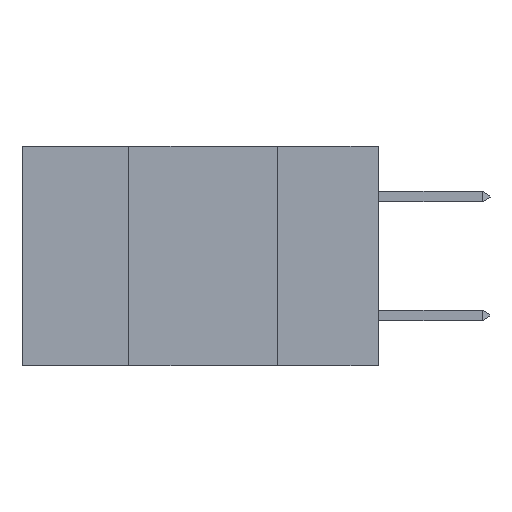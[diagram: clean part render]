
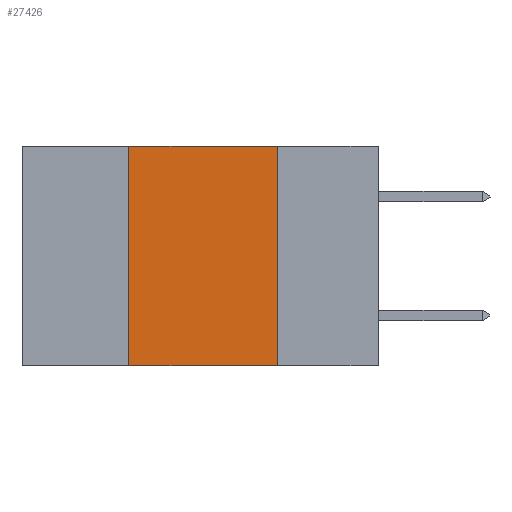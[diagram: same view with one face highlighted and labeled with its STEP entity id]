
A CAD part, left-side view. The second image highlights one B-rep face of the part: STEP entity #27426.
In plain terms, the highlighted planar face has unit normal (-1, 0, 0).
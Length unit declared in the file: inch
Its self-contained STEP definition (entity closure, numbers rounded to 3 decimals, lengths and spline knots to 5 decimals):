
#52 = CARTESIAN_POINT ( 'NONE',  ( 0., 0.17, 0. ) ) ;
#2374 = ORIENTED_EDGE ( 'NONE', *, *, #3231, .F. ) ;
#2716 = VERTEX_POINT ( 'NONE', #6277 ) ;
#2918 = DIRECTION ( 'NONE',  ( 0., -1., 0. ) ) ;
#3231 = EDGE_CURVE ( 'NONE', #17648, #2716, #27970, .T. ) ;
#6277 = CARTESIAN_POINT ( 'NONE',  ( 0., 0.42, 0. ) ) ;
#7443 = PLANE ( 'NONE',  #23308 ) ;
#7758 = EDGE_LOOP ( 'NONE', ( #9917, #26870, #2374, #13722 ) ) ;
#7793 = CARTESIAN_POINT ( 'NONE',  ( 0., 0.6, 0. ) ) ;
#8834 = VECTOR ( 'NONE', #10053, 39.37008 ) ;
#8847 = VECTOR ( 'NONE', #10106, 39.37008 ) ;
#9709 = DIRECTION ( 'NONE',  ( 1., 0., 0. ) ) ;
#9917 = ORIENTED_EDGE ( 'NONE', *, *, #11783, .F. ) ;
#10053 = DIRECTION ( 'NONE',  ( 0., -1., 0. ) ) ;
#10106 = DIRECTION ( 'NONE',  ( 0., 0., -1. ) ) ;
#10343 = DIRECTION ( 'NONE',  ( 0., 0., 1. ) ) ;
#11783 = EDGE_CURVE ( 'NONE', #18381, #17428, #20709, .T. ) ;
#13722 = ORIENTED_EDGE ( 'NONE', *, *, #20954, .T. ) ;
#14723 = LINE ( 'NONE', #25275, #19960 ) ;
#14748 = LINE ( 'NONE', #7793, #8834 ) ;
#17428 = VERTEX_POINT ( 'NONE', #23968 ) ;
#17648 = VERTEX_POINT ( 'NONE', #17990 ) ;
#17990 = CARTESIAN_POINT ( 'NONE',  ( 0., 0.42, -0.37 ) ) ;
#18381 = VERTEX_POINT ( 'NONE', #52 ) ;
#19960 = VECTOR ( 'NONE', #2918, 39.37008 ) ;
#20498 = EDGE_CURVE ( 'NONE', #2716, #18381, #14748, .T. ) ;
#20709 = LINE ( 'NONE', #23431, #8847 ) ;
#20954 = EDGE_CURVE ( 'NONE', #17648, #17428, #14723, .T. ) ;
#22195 = VECTOR ( 'NONE', #10343, 39.37008 ) ;
#23036 = CARTESIAN_POINT ( 'NONE',  ( 0., 0.6, 0. ) ) ;
#23308 = AXIS2_PLACEMENT_3D ( 'NONE', #23036, #9709, #25254 ) ;
#23431 = CARTESIAN_POINT ( 'NONE',  ( 0., 0.17, 0. ) ) ;
#23968 = CARTESIAN_POINT ( 'NONE',  ( 0., 0.17, -0.37 ) ) ;
#24233 = FACE_OUTER_BOUND ( 'NONE', #7758, .T. ) ;
#25254 = DIRECTION ( 'NONE',  ( 0., 0., -1. ) ) ;
#25275 = CARTESIAN_POINT ( 'NONE',  ( 0., 0.6, -0.37 ) ) ;
#26870 = ORIENTED_EDGE ( 'NONE', *, *, #20498, .F. ) ;
#27426 = ADVANCED_FACE ( 'NONE', ( #24233 ), #7443, .F. ) ;
#27970 = LINE ( 'NONE', #28177, #22195 ) ;
#28177 = CARTESIAN_POINT ( 'NONE',  ( 0., 0.42, 0. ) ) ;
